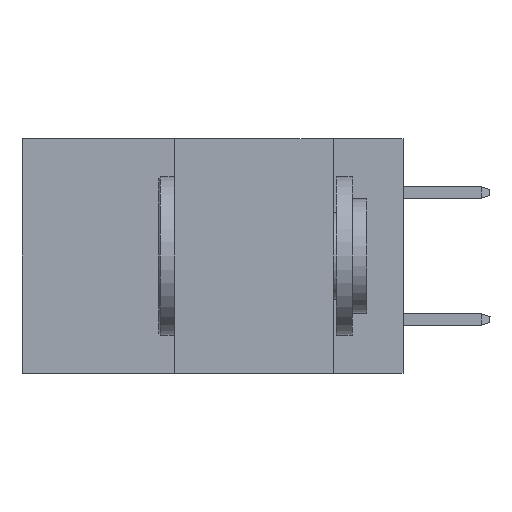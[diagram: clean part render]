
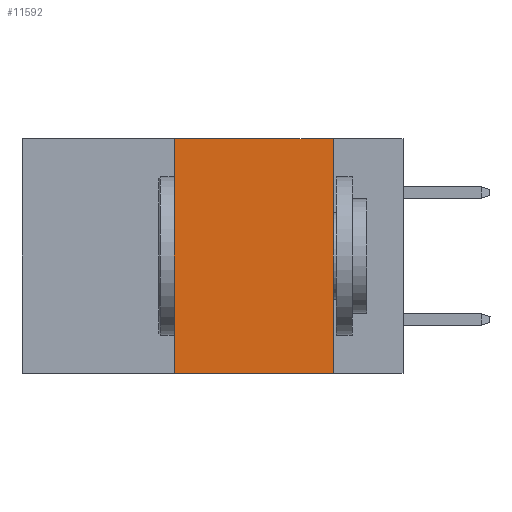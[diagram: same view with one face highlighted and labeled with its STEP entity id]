
A CAD part, left-side view. The second image highlights one B-rep face of the part: STEP entity #11592.
In plain terms, the highlighted planar face has unit normal (-1, 0, 0).
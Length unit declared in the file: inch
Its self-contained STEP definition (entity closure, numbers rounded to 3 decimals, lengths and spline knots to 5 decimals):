
#472 = FACE_OUTER_BOUND ( 'NONE', #22277, .T. ) ;
#560 = ORIENTED_EDGE ( 'NONE', *, *, #16453, .F. ) ;
#2883 = VERTEX_POINT ( 'NONE', #10123 ) ;
#2952 = EDGE_CURVE ( 'NONE', #29297, #25988, #27486, .T. ) ;
#3041 = DIRECTION ( 'NONE',  ( 0., 0., 1. ) ) ;
#3055 = CARTESIAN_POINT ( 'NONE',  ( 0., 0.11, 0. ) ) ;
#3206 = ORIENTED_EDGE ( 'NONE', *, *, #21316, .T. ) ;
#4045 = CARTESIAN_POINT ( 'NONE',  ( 0., 0.11, 0. ) ) ;
#4680 = PLANE ( 'NONE',  #8287 ) ;
#4998 = ORIENTED_EDGE ( 'NONE', *, *, #2952, .F. ) ;
#5962 = DIRECTION ( 'NONE',  ( 0., -1., 0. ) ) ;
#8287 = AXIS2_PLACEMENT_3D ( 'NONE', #14432, #26201, #23717 ) ;
#9426 = CARTESIAN_POINT ( 'NONE',  ( 0., 0.36, 0. ) ) ;
#9879 = DIRECTION ( 'NONE',  ( 0., 0., -1. ) ) ;
#10123 = CARTESIAN_POINT ( 'NONE',  ( 0., 0.36, -0.37 ) ) ;
#10321 = LINE ( 'NONE', #24273, #17538 ) ;
#10927 = DIRECTION ( 'NONE',  ( 0., -1., 0. ) ) ;
#11592 = ADVANCED_FACE ( 'NONE', ( #472 ), #4680, .F. ) ;
#13067 = CARTESIAN_POINT ( 'NONE',  ( 0., 0.6, 0. ) ) ;
#14432 = CARTESIAN_POINT ( 'NONE',  ( 0., 0.6, 0. ) ) ;
#14474 = VECTOR ( 'NONE', #10927, 39.37008 ) ;
#15295 = CARTESIAN_POINT ( 'NONE',  ( 0., 0.6, -0.37 ) ) ;
#16453 = EDGE_CURVE ( 'NONE', #25988, #24740, #28929, .T. ) ;
#17538 = VECTOR ( 'NONE', #3041, 39.37008 ) ;
#18717 = ORIENTED_EDGE ( 'NONE', *, *, #23213, .F. ) ;
#19814 = VECTOR ( 'NONE', #9879, 39.37008 ) ;
#19944 = LINE ( 'NONE', #15295, #14474 ) ;
#21316 = EDGE_CURVE ( 'NONE', #2883, #24740, #19944, .T. ) ;
#22277 = EDGE_LOOP ( 'NONE', ( #560, #4998, #18717, #3206 ) ) ;
#23213 = EDGE_CURVE ( 'NONE', #2883, #29297, #10321, .T. ) ;
#23717 = DIRECTION ( 'NONE',  ( 0., 0., -1. ) ) ;
#24273 = CARTESIAN_POINT ( 'NONE',  ( 0., 0.36, 0. ) ) ;
#24439 = VECTOR ( 'NONE', #5962, 39.37008 ) ;
#24740 = VERTEX_POINT ( 'NONE', #29680 ) ;
#25988 = VERTEX_POINT ( 'NONE', #4045 ) ;
#26201 = DIRECTION ( 'NONE',  ( 1., 0., 0. ) ) ;
#27486 = LINE ( 'NONE', #13067, #24439 ) ;
#28929 = LINE ( 'NONE', #3055, #19814 ) ;
#29297 = VERTEX_POINT ( 'NONE', #9426 ) ;
#29680 = CARTESIAN_POINT ( 'NONE',  ( 0., 0.11, -0.37 ) ) ;
